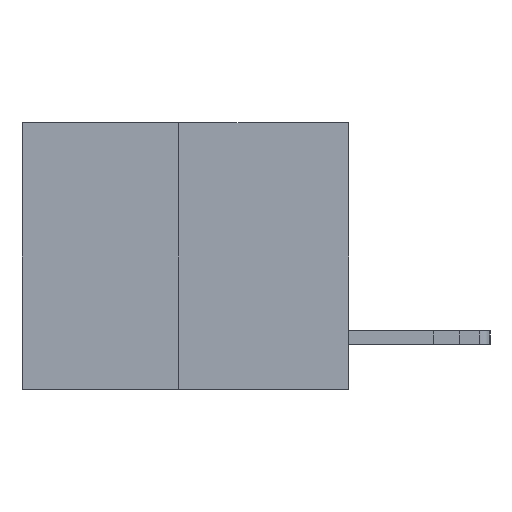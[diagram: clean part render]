
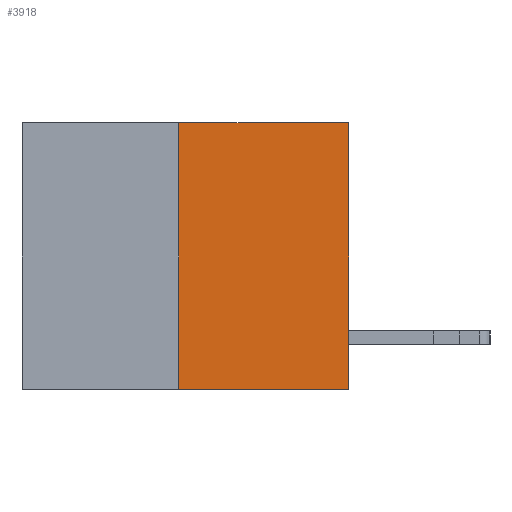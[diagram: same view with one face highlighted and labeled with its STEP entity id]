
A CAD part, left-side view. The second image highlights one B-rep face of the part: STEP entity #3918.
In plain terms, the highlighted planar face has unit normal (-1, 0, 0).
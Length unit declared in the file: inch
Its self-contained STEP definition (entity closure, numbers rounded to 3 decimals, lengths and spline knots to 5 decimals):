
#718 = VERTEX_POINT ( 'NONE', #800 ) ;
#800 = CARTESIAN_POINT ( 'NONE',  ( 0., 0., 0. ) ) ;
#1164 = DIRECTION ( 'NONE',  ( 0., 0., 1. ) ) ;
#1301 = EDGE_CURVE ( 'NONE', #16529, #718, #8580, .T. ) ;
#1456 = CARTESIAN_POINT ( 'NONE',  ( 0., 0.312, 0. ) ) ;
#1638 = ORIENTED_EDGE ( 'NONE', *, *, #17631, .F. ) ;
#1670 = CARTESIAN_POINT ( 'NONE',  ( 0., 0.6, -0.49 ) ) ;
#2375 = LINE ( 'NONE', #6991, #2595 ) ;
#2595 = VECTOR ( 'NONE', #15046, 39.37008 ) ;
#2762 = DIRECTION ( 'NONE',  ( 0., 0., -1. ) ) ;
#3060 = AXIS2_PLACEMENT_3D ( 'NONE', #9530, #8170, #2762 ) ;
#3918 = ADVANCED_FACE ( 'NONE', ( #3947 ), #4250, .F. ) ;
#3947 = FACE_OUTER_BOUND ( 'NONE', #6939, .T. ) ;
#4250 = PLANE ( 'NONE',  #3060 ) ;
#4270 = ORIENTED_EDGE ( 'NONE', *, *, #15311, .T. ) ;
#6939 = EDGE_LOOP ( 'NONE', ( #1638, #4270, #10290, #8463 ) ) ;
#6991 = CARTESIAN_POINT ( 'NONE',  ( 0., 0.6, 0. ) ) ;
#7697 = LINE ( 'NONE', #16388, #17080 ) ;
#8132 = VECTOR ( 'NONE', #1164, 39.37008 ) ;
#8170 = DIRECTION ( 'NONE',  ( 1., 0., 0. ) ) ;
#8452 = VERTEX_POINT ( 'NONE', #13765 ) ;
#8463 = ORIENTED_EDGE ( 'NONE', *, *, #13784, .F. ) ;
#8580 = LINE ( 'NONE', #12136, #8132 ) ;
#9530 = CARTESIAN_POINT ( 'NONE',  ( 0., 0.6, 0. ) ) ;
#10114 = VECTOR ( 'NONE', #14208, 39.37008 ) ;
#10290 = ORIENTED_EDGE ( 'NONE', *, *, #1301, .T. ) ;
#11503 = VERTEX_POINT ( 'NONE', #1456 ) ;
#12136 = CARTESIAN_POINT ( 'NONE',  ( 0., 0., 0. ) ) ;
#12927 = CARTESIAN_POINT ( 'NONE',  ( 0., 0., -0.49 ) ) ;
#13611 = DIRECTION ( 'NONE',  ( 0., 0., 1. ) ) ;
#13765 = CARTESIAN_POINT ( 'NONE',  ( 0., 0.312, -0.49 ) ) ;
#13780 = LINE ( 'NONE', #1670, #10114 ) ;
#13784 = EDGE_CURVE ( 'NONE', #11503, #718, #2375, .T. ) ;
#14208 = DIRECTION ( 'NONE',  ( 0., -1., 0. ) ) ;
#15046 = DIRECTION ( 'NONE',  ( 0., -1., 0. ) ) ;
#15311 = EDGE_CURVE ( 'NONE', #8452, #16529, #13780, .T. ) ;
#16388 = CARTESIAN_POINT ( 'NONE',  ( 0., 0.312, -0.49 ) ) ;
#16529 = VERTEX_POINT ( 'NONE', #12927 ) ;
#17080 = VECTOR ( 'NONE', #13611, 39.37008 ) ;
#17631 = EDGE_CURVE ( 'NONE', #8452, #11503, #7697, .T. ) ;
